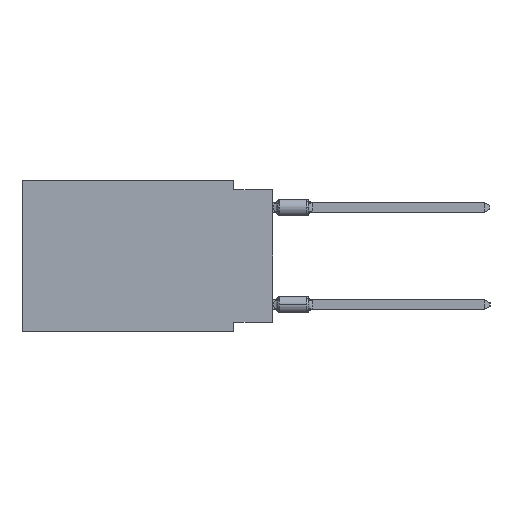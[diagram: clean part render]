
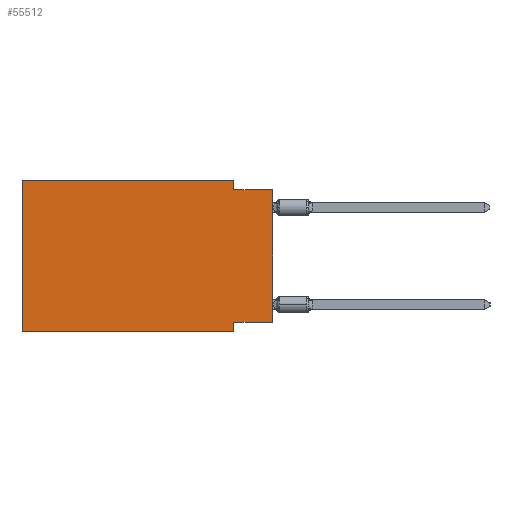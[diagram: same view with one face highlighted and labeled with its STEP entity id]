
A CAD part, left-side view. The second image highlights one B-rep face of the part: STEP entity #55512.
In plain terms, the highlighted planar face has unit normal (-1, 0, 0).
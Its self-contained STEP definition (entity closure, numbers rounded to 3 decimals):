
#125 = VECTOR ( 'NONE', #3471, 1000. ) ;
#474 = CARTESIAN_POINT ( 'NONE',  ( 0., 0., 0. ) ) ;
#3325 = VECTOR ( 'NONE', #31653, 1000. ) ;
#3471 = DIRECTION ( 'NONE',  ( 0., 1., 0. ) ) ;
#4115 = ORIENTED_EDGE ( 'NONE', *, *, #50987, .T. ) ;
#4468 = VECTOR ( 'NONE', #37539, 1000. ) ;
#4582 = CARTESIAN_POINT ( 'NONE',  ( 0., 16.383, 0. ) ) ;
#5569 = EDGE_CURVE ( 'NONE', #6374, #31114, #26452, .T. ) ;
#5584 = VECTOR ( 'NONE', #53083, 1000. ) ;
#5689 = AXIS2_PLACEMENT_3D ( 'NONE', #31201, #22640, #40045 ) ;
#6374 = VERTEX_POINT ( 'NONE', #48279 ) ;
#8161 = LINE ( 'NONE', #42996, #50014 ) ;
#8925 = DIRECTION ( 'NONE',  ( 0., -1., 0. ) ) ;
#11179 = CARTESIAN_POINT ( 'NONE',  ( 0., 16.383, -9.906 ) ) ;
#12652 = LINE ( 'NONE', #43189, #21715 ) ;
#13008 = ORIENTED_EDGE ( 'NONE', *, *, #30143, .F. ) ;
#13477 = DIRECTION ( 'NONE',  ( 0., 0., -1. ) ) ;
#14822 = ORIENTED_EDGE ( 'NONE', *, *, #30239, .F. ) ;
#16039 = LINE ( 'NONE', #16881, #125 ) ;
#16834 = EDGE_CURVE ( 'NONE', #50502, #31114, #47766, .T. ) ;
#16881 = CARTESIAN_POINT ( 'NONE',  ( 0., 0., -9.271 ) ) ;
#17013 = DIRECTION ( 'NONE',  ( 0., -1., 0. ) ) ;
#17882 = DIRECTION ( 'NONE',  ( 0., 0., 1. ) ) ;
#18071 = EDGE_LOOP ( 'NONE', ( #21777, #54433, #39281, #36491, #14822, #4115, #21846, #13008 ) ) ;
#18357 = PLANE ( 'NONE',  #5689 ) ;
#19297 = EDGE_CURVE ( 'NONE', #19944, #51929, #8161, .T. ) ;
#19944 = VERTEX_POINT ( 'NONE', #41723 ) ;
#21142 = VERTEX_POINT ( 'NONE', #11179 ) ;
#21715 = VECTOR ( 'NONE', #13477, 1000. ) ;
#21777 = ORIENTED_EDGE ( 'NONE', *, *, #5569, .T. ) ;
#21846 = ORIENTED_EDGE ( 'NONE', *, *, #47642, .F. ) ;
#22357 = FACE_OUTER_BOUND ( 'NONE', #18071, .T. ) ;
#22640 = DIRECTION ( 'NONE',  ( 1., 0., 0. ) ) ;
#26452 = LINE ( 'NONE', #474, #55566 ) ;
#28102 = CARTESIAN_POINT ( 'NONE',  ( 0., 2.54, -9.271 ) ) ;
#28417 = CARTESIAN_POINT ( 'NONE',  ( 0., 16.383, -9.906 ) ) ;
#28455 = CARTESIAN_POINT ( 'NONE',  ( 0., 2.54, -9.906 ) ) ;
#30143 = EDGE_CURVE ( 'NONE', #6374, #32504, #16039, .T. ) ;
#30239 = EDGE_CURVE ( 'NONE', #21142, #19944, #39409, .T. ) ;
#30895 = VERTEX_POINT ( 'NONE', #28455 ) ;
#31114 = VERTEX_POINT ( 'NONE', #47542 ) ;
#31201 = CARTESIAN_POINT ( 'NONE',  ( 0., 16.383, 0. ) ) ;
#31653 = DIRECTION ( 'NONE',  ( 0., 0., -1. ) ) ;
#32504 = VERTEX_POINT ( 'NONE', #28102 ) ;
#36491 = ORIENTED_EDGE ( 'NONE', *, *, #19297, .F. ) ;
#37061 = LINE ( 'NONE', #54188, #3325 ) ;
#37539 = DIRECTION ( 'NONE',  ( 0., -1., 0. ) ) ;
#39202 = CARTESIAN_POINT ( 'NONE',  ( 0., 0., -0.635 ) ) ;
#39281 = ORIENTED_EDGE ( 'NONE', *, *, #49987, .F. ) ;
#39409 = LINE ( 'NONE', #4582, #5584 ) ;
#40045 = DIRECTION ( 'NONE',  ( 0., 0., -1. ) ) ;
#41723 = CARTESIAN_POINT ( 'NONE',  ( 0., 16.383, 0. ) ) ;
#42996 = CARTESIAN_POINT ( 'NONE',  ( 0., 16.383, 0. ) ) ;
#43189 = CARTESIAN_POINT ( 'NONE',  ( 0., 2.54, 0. ) ) ;
#43297 = CARTESIAN_POINT ( 'NONE',  ( 0., 2.54, 0. ) ) ;
#45893 = CARTESIAN_POINT ( 'NONE',  ( 0., 2.54, -0.635 ) ) ;
#47542 = CARTESIAN_POINT ( 'NONE',  ( 0., 0., -0.635 ) ) ;
#47642 = EDGE_CURVE ( 'NONE', #32504, #30895, #37061, .T. ) ;
#47766 = LINE ( 'NONE', #39202, #53479 ) ;
#48279 = CARTESIAN_POINT ( 'NONE',  ( 0., 0., -9.271 ) ) ;
#49987 = EDGE_CURVE ( 'NONE', #51929, #50502, #12652, .T. ) ;
#50014 = VECTOR ( 'NONE', #17013, 1000. ) ;
#50093 = LINE ( 'NONE', #28417, #4468 ) ;
#50502 = VERTEX_POINT ( 'NONE', #45893 ) ;
#50987 = EDGE_CURVE ( 'NONE', #21142, #30895, #50093, .T. ) ;
#51929 = VERTEX_POINT ( 'NONE', #43297 ) ;
#53083 = DIRECTION ( 'NONE',  ( 0., 0., 1. ) ) ;
#53479 = VECTOR ( 'NONE', #8925, 1000. ) ;
#54188 = CARTESIAN_POINT ( 'NONE',  ( 0., 2.54, -9.906 ) ) ;
#54433 = ORIENTED_EDGE ( 'NONE', *, *, #16834, .F. ) ;
#55512 = ADVANCED_FACE ( 'NONE', ( #22357 ), #18357, .F. ) ;
#55566 = VECTOR ( 'NONE', #17882, 1000. ) ;
